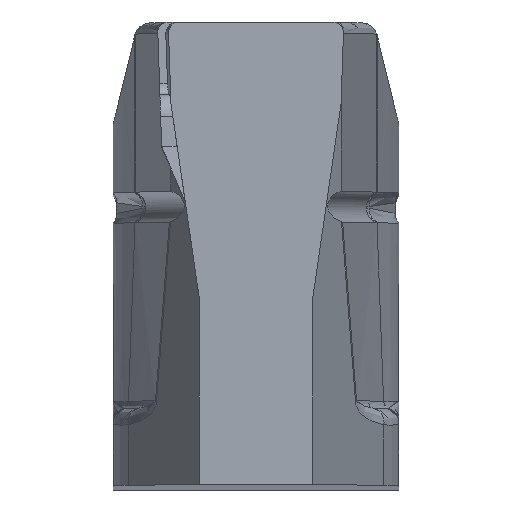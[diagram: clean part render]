
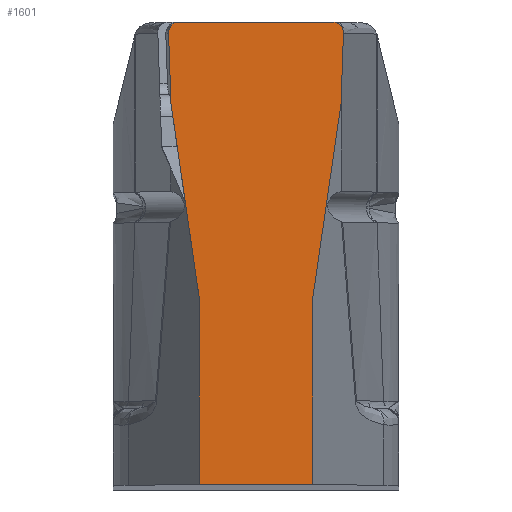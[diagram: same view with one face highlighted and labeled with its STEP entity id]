
A CAD part, top view. The second image highlights one B-rep face of the part: STEP entity #1601.
In plain terms, the highlighted planar face has unit normal (0, 0, 1).
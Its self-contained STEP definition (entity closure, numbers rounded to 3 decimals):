
#48=ELLIPSE('',#1727,0.691,0.689);
#49=ELLIPSE('',#1729,0.691,0.689);
#259=FACE_OUTER_BOUND('',#350,.T.);
#350=EDGE_LOOP('',(#1469,#1470,#1471,#1472,#1473,#1474,#1475,#1476,#1477,
#1478));
#388=LINE('',#2417,#495);
#393=LINE('',#2426,#500);
#446=LINE('',#4259,#553);
#448=LINE('',#4289,#555);
#451=LINE('',#4320,#558);
#453=LINE('',#4324,#560);
#455=LINE('',#4328,#562);
#457=LINE('',#4331,#564);
#495=VECTOR('',#1812,10.);
#500=VECTOR('',#1819,10.);
#553=VECTOR('',#2054,10.);
#555=VECTOR('',#2060,10.);
#558=VECTOR('',#2067,10.);
#560=VECTOR('',#2071,10.);
#562=VECTOR('',#2075,10.);
#564=VECTOR('',#2079,10.);
#647=VERTEX_POINT('',#2414);
#648=VERTEX_POINT('',#2416);
#651=VERTEX_POINT('',#2424);
#749=VERTEX_POINT('',#4257);
#750=VERTEX_POINT('',#4284);
#751=VERTEX_POINT('',#4288);
#752=VERTEX_POINT('',#4315);
#753=VERTEX_POINT('',#4319);
#754=VERTEX_POINT('',#4323);
#755=VERTEX_POINT('',#4327);
#811=EDGE_CURVE('',#648,#647,#388,.T.);
#816=EDGE_CURVE('',#647,#651,#393,.T.);
#983=EDGE_CURVE('',#651,#749,#446,.T.);
#984=EDGE_CURVE('',#750,#648,#48,.T.);
#986=EDGE_CURVE('',#751,#750,#448,.T.);
#988=EDGE_CURVE('',#752,#751,#49,.T.);
#990=EDGE_CURVE('',#753,#752,#451,.T.);
#992=EDGE_CURVE('',#754,#753,#453,.T.);
#994=EDGE_CURVE('',#755,#754,#455,.T.);
#996=EDGE_CURVE('',#749,#755,#457,.T.);
#1469=ORIENTED_EDGE('',*,*,#996,.T.);
#1470=ORIENTED_EDGE('',*,*,#994,.T.);
#1471=ORIENTED_EDGE('',*,*,#992,.T.);
#1472=ORIENTED_EDGE('',*,*,#990,.T.);
#1473=ORIENTED_EDGE('',*,*,#988,.T.);
#1474=ORIENTED_EDGE('',*,*,#986,.T.);
#1475=ORIENTED_EDGE('',*,*,#984,.T.);
#1476=ORIENTED_EDGE('',*,*,#811,.T.);
#1477=ORIENTED_EDGE('',*,*,#816,.T.);
#1478=ORIENTED_EDGE('',*,*,#983,.T.);
#1510=PLANE('',#1734);
#1601=ADVANCED_FACE('',(#259),#1510,.T.);
#1727=AXIS2_PLACEMENT_3D('',#4285,#2055,#2056);
#1729=AXIS2_PLACEMENT_3D('',#4316,#2062,#2063);
#1734=AXIS2_PLACEMENT_3D('',#4332,#2080,#2081);
#1812=DIRECTION('',(0.034,-0.999,0.));
#1819=DIRECTION('',(0.144,-0.99,0.));
#2054=DIRECTION('',(0.,-1.,0.));
#2055=DIRECTION('center_axis',(0.,0.,
1.));
#2056=DIRECTION('ref_axis',(1.,0.,0.));
#2060=DIRECTION('',(-1.,0.,0.));
#2062=DIRECTION('center_axis',(0.,0.,1.));
#2063=DIRECTION('ref_axis',(1.,0.,0.));
#2067=DIRECTION('',(0.034,0.999,0.));
#2071=DIRECTION('',(0.144,0.99,0.));
#2075=DIRECTION('',(0.,1.,0.));
#2079=DIRECTION('',(1.,0.,0.));
#2080=DIRECTION('center_axis',(0.,0.,1.));
#2081=DIRECTION('ref_axis',(1.,0.,0.));
#2414=CARTESIAN_POINT('',(-5.572,9.684,153.212));
#2416=CARTESIAN_POINT('',(-5.724,14.215,153.212));
#2417=CARTESIAN_POINT('',(-5.311,1.913,153.212));
#2424=CARTESIAN_POINT('',(-3.753,-2.837,153.212));
#2426=CARTESIAN_POINT('',(-3.628,-3.702,153.212));
#4257=CARTESIAN_POINT('',(-3.753,-14.872,153.212));
#4259=CARTESIAN_POINT('',(-3.753,-8.091,153.212));
#4284=CARTESIAN_POINT('',(-5.034,14.927,153.212));
#4285=CARTESIAN_POINT('Origin',(-5.034,14.238,153.212));
#4288=CARTESIAN_POINT('',(4.853,14.927,153.212));
#4289=CARTESIAN_POINT('',(7.829,14.927,153.212));
#4315=CARTESIAN_POINT('',(5.543,14.215,153.212));
#4316=CARTESIAN_POINT('Origin',(4.853,14.238,153.212));
#4319=CARTESIAN_POINT('',(5.391,9.684,153.212));
#4320=CARTESIAN_POINT('',(5.13,1.913,153.212));
#4323=CARTESIAN_POINT('',(3.573,-2.837,153.212));
#4324=CARTESIAN_POINT('',(3.447,-3.702,153.212));
#4327=CARTESIAN_POINT('',(3.573,-14.872,153.212));
#4328=CARTESIAN_POINT('',(3.573,-8.091,153.212));
#4331=CARTESIAN_POINT('',(0.107,-14.872,153.212));
#4332=CARTESIAN_POINT('Origin',(-0.091,-0.121,
153.212));
